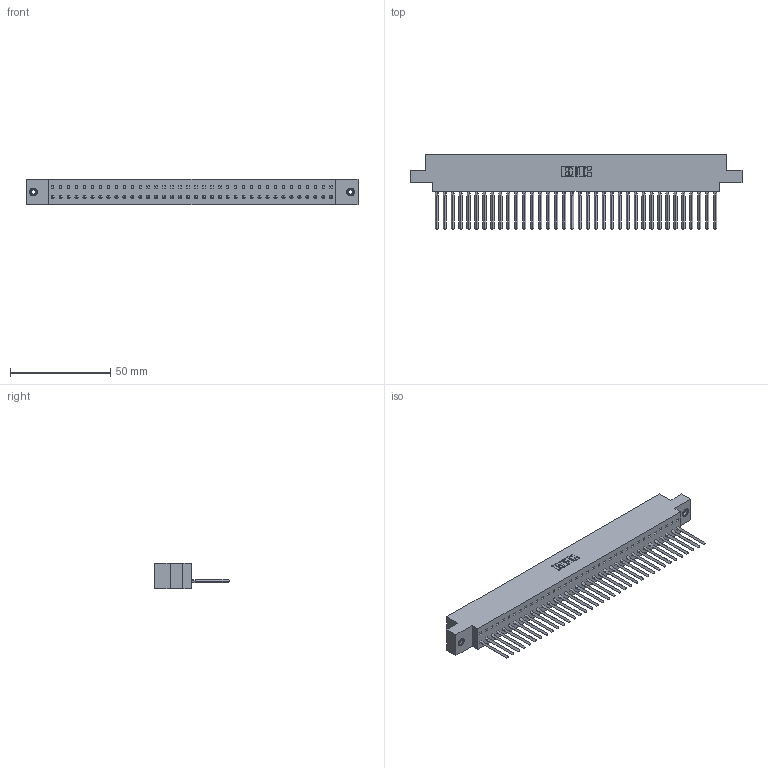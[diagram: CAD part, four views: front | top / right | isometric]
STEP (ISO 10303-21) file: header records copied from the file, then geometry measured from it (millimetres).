
FILE_DESCRIPTION (( 'STEP AP203' ), '1' );
FILE_NAME ('317-036-541-678.STEP', '2020-02-27T22:41:45', ( '' ), ( '' ), 'SwSTEP 2.0', 'SolidWorks 2016', '' );
FILE_SCHEMA (( 'CONFIG_CONTROL_DESIGN' ));
Length unit declared in the file: inch
Products named in the file (4): 317-036-541-678; 317 Part_.156 Dia - TI; 317-290-002_541; 345-250-001_345-250-003-102
Assembly tree (39 placements, depth 2):
  317-036-541-678
    317 Part_.156 Dia - TI
    317-290-002_541  x36
    345-250-001_345-250-003-102  x2
Bounding box: 165.35 x 37.34 x 12.7 mm (x, y, z)
Volume: 26623.9 mm3; surface area: 37442.8 mm2
Topology: 39 solids, 39 shells, 5634 faces, 16035 edges, 10418 vertices
Faces by surface type: plane 4554, cylinder 920, bspline 144, cone 12, torus 4
Entity records: 54457 total; most frequent: CARTESIAN_POINT 10288, ORIENTED_EDGE 9570, DIRECTION 7899, EDGE_CURVE 4785, LINE 4401, VECTOR 4401, VERTEX_POINT 3178, AXIS2_PLACEMENT_3D 1749
